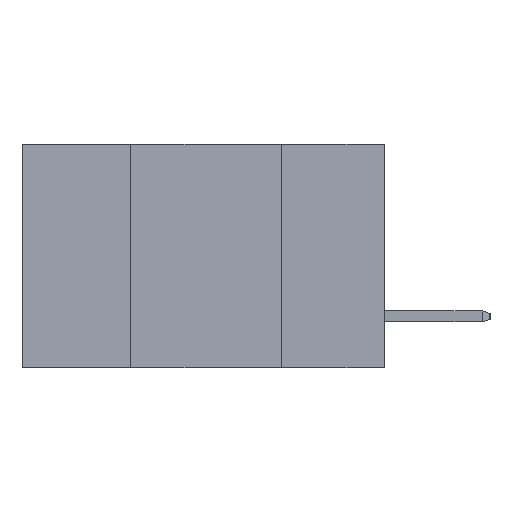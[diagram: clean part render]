
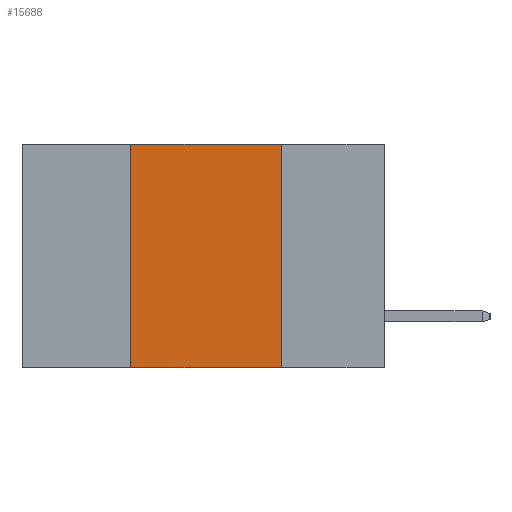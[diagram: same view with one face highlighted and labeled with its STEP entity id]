
A CAD part, left-side view. The second image highlights one B-rep face of the part: STEP entity #15688.
In plain terms, the highlighted planar face has unit normal (-1, 0, 0).
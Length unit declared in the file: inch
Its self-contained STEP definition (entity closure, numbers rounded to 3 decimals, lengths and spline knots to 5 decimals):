
#327 = CARTESIAN_POINT ( 'NONE',  ( 0., 0.6, 0. ) ) ;
#757 = CARTESIAN_POINT ( 'NONE',  ( 0., 0.42, 0. ) ) ;
#1157 = VERTEX_POINT ( 'NONE', #18911 ) ;
#2652 = CARTESIAN_POINT ( 'NONE',  ( 0., 0.6, 0. ) ) ;
#2790 = DIRECTION ( 'NONE',  ( 1., 0., 0. ) ) ;
#3024 = EDGE_CURVE ( 'NONE', #1157, #3470, #30703, .T. ) ;
#3470 = VERTEX_POINT ( 'NONE', #757 ) ;
#5569 = VECTOR ( 'NONE', #20784, 39.37008 ) ;
#6298 = CARTESIAN_POINT ( 'NONE',  ( 0., 0.17, 0. ) ) ;
#7549 = DIRECTION ( 'NONE',  ( 0., -1., 0. ) ) ;
#8845 = ORIENTED_EDGE ( 'NONE', *, *, #9562, .T. ) ;
#9562 = EDGE_CURVE ( 'NONE', #1157, #13233, #20283, .T. ) ;
#10361 = ORIENTED_EDGE ( 'NONE', *, *, #3024, .F. ) ;
#10882 = EDGE_CURVE ( 'NONE', #3470, #18458, #19886, .T. ) ;
#11107 = ORIENTED_EDGE ( 'NONE', *, *, #10882, .F. ) ;
#13233 = VERTEX_POINT ( 'NONE', #16862 ) ;
#13488 = CARTESIAN_POINT ( 'NONE',  ( 0., 0.42, 0. ) ) ;
#14885 = PLANE ( 'NONE',  #15863 ) ;
#15688 = ADVANCED_FACE ( 'NONE', ( #19966 ), #14885, .F. ) ;
#15863 = AXIS2_PLACEMENT_3D ( 'NONE', #327, #2790, #19688 ) ;
#16395 = CARTESIAN_POINT ( 'NONE',  ( 0., 0.17, 0. ) ) ;
#16478 = EDGE_LOOP ( 'NONE', ( #29857, #11107, #10361, #8845 ) ) ;
#16862 = CARTESIAN_POINT ( 'NONE',  ( 0., 0.17, -0.37 ) ) ;
#17168 = DIRECTION ( 'NONE',  ( 0., -1., 0. ) ) ;
#17746 = LINE ( 'NONE', #16395, #23228 ) ;
#18458 = VERTEX_POINT ( 'NONE', #6298 ) ;
#18911 = CARTESIAN_POINT ( 'NONE',  ( 0., 0.42, -0.37 ) ) ;
#19688 = DIRECTION ( 'NONE',  ( 0., 0., -1. ) ) ;
#19886 = LINE ( 'NONE', #2652, #25318 ) ;
#19966 = FACE_OUTER_BOUND ( 'NONE', #16478, .T. ) ;
#20283 = LINE ( 'NONE', #21869, #27896 ) ;
#20784 = DIRECTION ( 'NONE',  ( 0., 0., 1. ) ) ;
#21869 = CARTESIAN_POINT ( 'NONE',  ( 0., 0.6, -0.37 ) ) ;
#23228 = VECTOR ( 'NONE', #23494, 39.37008 ) ;
#23494 = DIRECTION ( 'NONE',  ( 0., 0., -1. ) ) ;
#25318 = VECTOR ( 'NONE', #17168, 39.37008 ) ;
#27896 = VECTOR ( 'NONE', #7549, 39.37008 ) ;
#28146 = EDGE_CURVE ( 'NONE', #18458, #13233, #17746, .T. ) ;
#29857 = ORIENTED_EDGE ( 'NONE', *, *, #28146, .F. ) ;
#30703 = LINE ( 'NONE', #13488, #5569 ) ;
